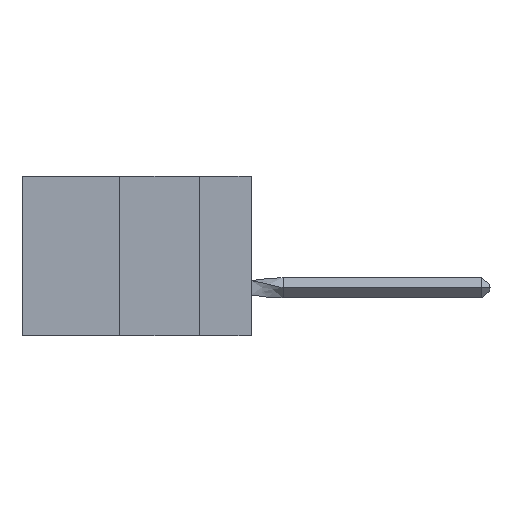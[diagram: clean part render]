
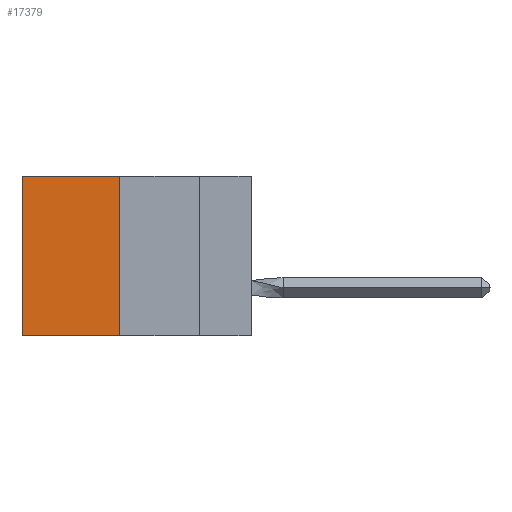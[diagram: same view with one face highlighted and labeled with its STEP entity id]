
A CAD part, left-side view. The second image highlights one B-rep face of the part: STEP entity #17379.
In plain terms, the highlighted planar face has unit normal (-1, 0, 0).
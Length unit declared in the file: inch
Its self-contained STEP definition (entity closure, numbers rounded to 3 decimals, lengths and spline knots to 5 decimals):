
#1309 = LINE ( 'NONE', #2179, #7334 ) ;
#2179 = CARTESIAN_POINT ( 'NONE',  ( 0.305, 0.413, 0. ) ) ;
#2917 = PLANE ( 'NONE',  #17937 ) ;
#3174 = CARTESIAN_POINT ( 'NONE',  ( 0.305, 0.413, -0.5 ) ) ;
#5590 = ORIENTED_EDGE ( 'NONE', *, *, #19490, .T. ) ;
#6027 = EDGE_LOOP ( 'NONE', ( #18720, #40768, #13069, #5590 ) ) ;
#7334 = VECTOR ( 'NONE', #36043, 39.37008 ) ;
#8471 = VECTOR ( 'NONE', #19656, 39.37008 ) ;
#9318 = CARTESIAN_POINT ( 'NONE',  ( 0.305, 0.72, -0.5 ) ) ;
#10714 = DIRECTION ( 'NONE',  ( 0., 0., -1. ) ) ;
#13069 = ORIENTED_EDGE ( 'NONE', *, *, #20107, .F. ) ;
#13910 = CARTESIAN_POINT ( 'NONE',  ( 0.305, 0.413, -0.5 ) ) ;
#17379 = ADVANCED_FACE ( 'NONE', ( #24395 ), #2917, .F. ) ;
#17937 = AXIS2_PLACEMENT_3D ( 'NONE', #3174, #25381, #25670 ) ;
#18301 = LINE ( 'NONE', #26854, #35403 ) ;
#18720 = ORIENTED_EDGE ( 'NONE', *, *, #28303, .T. ) ;
#19490 = EDGE_CURVE ( 'NONE', #34061, #25146, #1309, .T. ) ;
#19656 = DIRECTION ( 'NONE',  ( 0., 1., 0. ) ) ;
#20107 = EDGE_CURVE ( 'NONE', #34061, #35151, #18301, .T. ) ;
#20882 = CARTESIAN_POINT ( 'NONE',  ( 0.305, 0.413, -0.5 ) ) ;
#20960 = VERTEX_POINT ( 'NONE', #9318 ) ;
#23796 = CARTESIAN_POINT ( 'NONE',  ( 0.305, 0.413, 0. ) ) ;
#24395 = FACE_OUTER_BOUND ( 'NONE', #6027, .T. ) ;
#25146 = VERTEX_POINT ( 'NONE', #40616 ) ;
#25381 = DIRECTION ( 'NONE',  ( 1., 0., 0. ) ) ;
#25670 = DIRECTION ( 'NONE',  ( 0., 0., -1. ) ) ;
#26854 = CARTESIAN_POINT ( 'NONE',  ( 0.305, 0.413, -0.5 ) ) ;
#28303 = EDGE_CURVE ( 'NONE', #25146, #20960, #29118, .T. ) ;
#29118 = LINE ( 'NONE', #29474, #39682 ) ;
#29474 = CARTESIAN_POINT ( 'NONE',  ( 0.305, 0.72, -0.5 ) ) ;
#32570 = DIRECTION ( 'NONE',  ( 0., 0., -1. ) ) ;
#33113 = LINE ( 'NONE', #13910, #8471 ) ;
#34061 = VERTEX_POINT ( 'NONE', #23796 ) ;
#35151 = VERTEX_POINT ( 'NONE', #20882 ) ;
#35403 = VECTOR ( 'NONE', #10714, 39.37008 ) ;
#36043 = DIRECTION ( 'NONE',  ( 0., 1., 0. ) ) ;
#38953 = EDGE_CURVE ( 'NONE', #35151, #20960, #33113, .T. ) ;
#39682 = VECTOR ( 'NONE', #32570, 39.37008 ) ;
#40616 = CARTESIAN_POINT ( 'NONE',  ( 0.305, 0.72, 0. ) ) ;
#40768 = ORIENTED_EDGE ( 'NONE', *, *, #38953, .F. ) ;
